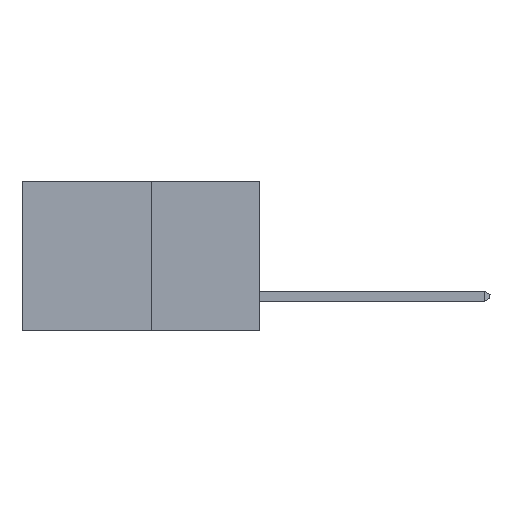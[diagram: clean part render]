
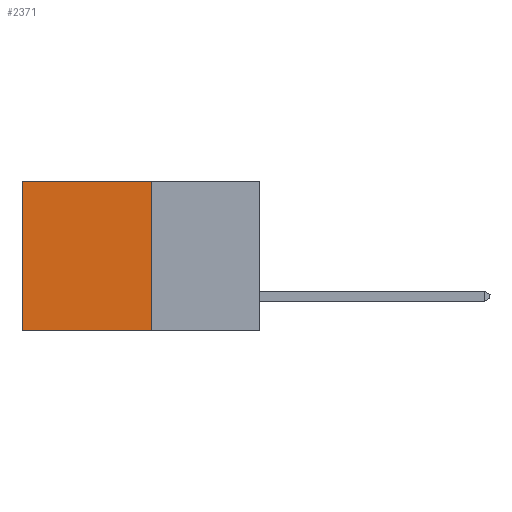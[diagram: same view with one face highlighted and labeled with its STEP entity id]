
A CAD part, left-side view. The second image highlights one B-rep face of the part: STEP entity #2371.
In plain terms, the highlighted planar face has unit normal (-1, 0, 0).
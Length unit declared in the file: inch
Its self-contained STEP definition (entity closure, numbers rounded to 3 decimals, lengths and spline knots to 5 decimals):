
#205 = EDGE_CURVE ( 'NONE', #7429, #4818, #10729, .T. ) ;
#597 = VERTEX_POINT ( 'NONE', #2857 ) ;
#668 = CARTESIAN_POINT ( 'NONE',  ( 0.277, 0.27, -0.37 ) ) ;
#1717 = ORIENTED_EDGE ( 'NONE', *, *, #2755, .F. ) ;
#2128 = DIRECTION ( 'NONE',  ( 0., 1., 0. ) ) ;
#2365 = ORIENTED_EDGE ( 'NONE', *, *, #9425, .T. ) ;
#2371 = ADVANCED_FACE ( 'NONE', ( #2658 ), #5708, .F. ) ;
#2539 = CARTESIAN_POINT ( 'NONE',  ( 0.277, 0.27, 0. ) ) ;
#2593 = CARTESIAN_POINT ( 'NONE',  ( 0.277, 0.27, -0.37 ) ) ;
#2658 = FACE_OUTER_BOUND ( 'NONE', #4885, .T. ) ;
#2755 = EDGE_CURVE ( 'NONE', #7226, #597, #8097, .T. ) ;
#2857 = CARTESIAN_POINT ( 'NONE',  ( 0.277, 0.59, -0.37 ) ) ;
#3000 = VECTOR ( 'NONE', #5309, 39.37008 ) ;
#4117 = ORIENTED_EDGE ( 'NONE', *, *, #205, .T. ) ;
#4449 = EDGE_CURVE ( 'NONE', #7429, #7226, #9340, .T. ) ;
#4490 = VECTOR ( 'NONE', #10622, 39.37008 ) ;
#4710 = ORIENTED_EDGE ( 'NONE', *, *, #4449, .F. ) ;
#4818 = VERTEX_POINT ( 'NONE', #7420 ) ;
#4885 = EDGE_LOOP ( 'NONE', ( #2365, #1717, #4710, #4117 ) ) ;
#5309 = DIRECTION ( 'NONE',  ( 0., 0., -1. ) ) ;
#5618 = CARTESIAN_POINT ( 'NONE',  ( 0.277, 0.59, -0.37 ) ) ;
#5708 = PLANE ( 'NONE',  #6736 ) ;
#6736 = AXIS2_PLACEMENT_3D ( 'NONE', #9717, #6884, #7639 ) ;
#6884 = DIRECTION ( 'NONE',  ( 1., 0., 0. ) ) ;
#7030 = CARTESIAN_POINT ( 'NONE',  ( 0.277, 0.27, -0.37 ) ) ;
#7226 = VERTEX_POINT ( 'NONE', #7030 ) ;
#7239 = CARTESIAN_POINT ( 'NONE',  ( 0.277, 0.27, 0. ) ) ;
#7356 = DIRECTION ( 'NONE',  ( 0., 1., 0. ) ) ;
#7420 = CARTESIAN_POINT ( 'NONE',  ( 0.277, 0.59, 0. ) ) ;
#7429 = VERTEX_POINT ( 'NONE', #2539 ) ;
#7639 = DIRECTION ( 'NONE',  ( 0., 0., -1. ) ) ;
#8097 = LINE ( 'NONE', #668, #10046 ) ;
#8547 = VECTOR ( 'NONE', #7356, 39.37008 ) ;
#9340 = LINE ( 'NONE', #2593, #3000 ) ;
#9425 = EDGE_CURVE ( 'NONE', #4818, #597, #10927, .T. ) ;
#9717 = CARTESIAN_POINT ( 'NONE',  ( 0.277, 0.27, -0.37 ) ) ;
#10046 = VECTOR ( 'NONE', #2128, 39.37008 ) ;
#10622 = DIRECTION ( 'NONE',  ( 0., 0., -1. ) ) ;
#10729 = LINE ( 'NONE', #7239, #8547 ) ;
#10927 = LINE ( 'NONE', #5618, #4490 ) ;
